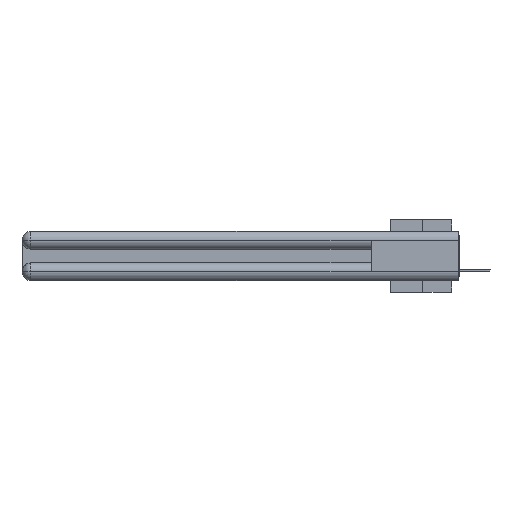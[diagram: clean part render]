
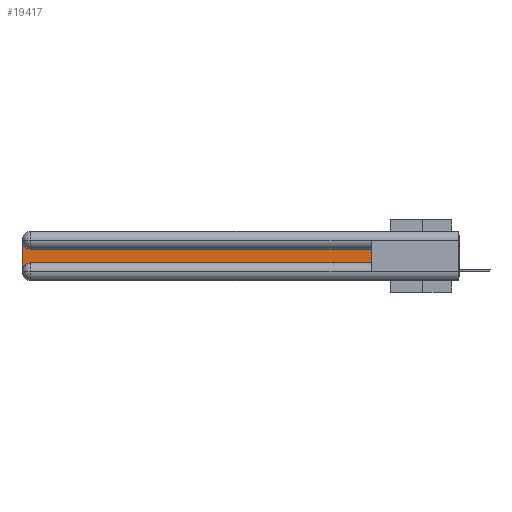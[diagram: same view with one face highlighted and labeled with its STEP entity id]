
A CAD part, left-side view. The second image highlights one B-rep face of the part: STEP entity #19417.
In plain terms, the highlighted planar face has unit normal (-1, 0, 0).
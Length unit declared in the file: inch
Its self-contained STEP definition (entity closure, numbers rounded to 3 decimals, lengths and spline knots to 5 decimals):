
#519 = FACE_OUTER_BOUND ( 'NONE', #23356, .T. ) ;
#742 = CARTESIAN_POINT ( 'NONE',  ( 0.075, 2.94, -0.2175 ) ) ;
#866 = EDGE_CURVE ( 'NONE', #18153, #22871, #3289, .T. ) ;
#1136 = VERTEX_POINT ( 'NONE', #16939 ) ;
#1238 = EDGE_CURVE ( 'NONE', #1136, #14046, #23736, .T. ) ;
#2180 = CARTESIAN_POINT ( 'NONE',  ( 0.075, 0.6, -0.2175 ) ) ;
#2908 = ORIENTED_EDGE ( 'NONE', *, *, #7068, .T. ) ;
#3167 = LINE ( 'NONE', #16044, #13963 ) ;
#3289 = LINE ( 'NONE', #4976, #29496 ) ;
#3975 = CARTESIAN_POINT ( 'NONE',  ( 0.075, 3., -0.0625 ) ) ;
#4450 = VERTEX_POINT ( 'NONE', #3975 ) ;
#4482 = VECTOR ( 'NONE', #19351, 39.37008 ) ;
#4976 = CARTESIAN_POINT ( 'NONE',  ( 0.075, 0.6, -0.2175 ) ) ;
#5127 = CARTESIAN_POINT ( 'NONE',  ( 0.075, 2.94, -0.1225 ) ) ;
#5492 = ORIENTED_EDGE ( 'NONE', *, *, #1238, .T. ) ;
#6933 = ORIENTED_EDGE ( 'NONE', *, *, #866, .T. ) ;
#7068 = EDGE_CURVE ( 'NONE', #4450, #1136, #25303, .T. ) ;
#7248 = AXIS2_PLACEMENT_3D ( 'NONE', #15810, #22698, #15716 ) ;
#7595 = DIRECTION ( 'NONE',  ( 0., -1., 0. ) ) ;
#10339 = CARTESIAN_POINT ( 'NONE',  ( 0.075, 3., -0.2175 ) ) ;
#10542 = CARTESIAN_POINT ( 'NONE',  ( 0.075, 0.6, -0.1225 ) ) ;
#10583 = VERTEX_POINT ( 'NONE', #5127 ) ;
#11145 = EDGE_CURVE ( 'NONE', #14046, #18153, #12526, .T. ) ;
#12526 = LINE ( 'NONE', #19443, #23641 ) ;
#12702 = AXIS2_PLACEMENT_3D ( 'NONE', #24027, #14924, #15028 ) ;
#13338 = CIRCLE ( 'NONE', #24314, 0.06 ) ;
#13963 = VECTOR ( 'NONE', #18340, 39.37008 ) ;
#14046 = VERTEX_POINT ( 'NONE', #742 ) ;
#14924 = DIRECTION ( 'NONE',  ( 1., 0., 0. ) ) ;
#15028 = DIRECTION ( 'NONE',  ( 0., 0., -1. ) ) ;
#15716 = DIRECTION ( 'NONE',  ( 0., 0., -1. ) ) ;
#15810 = CARTESIAN_POINT ( 'NONE',  ( 0.075, 3., -0.1225 ) ) ;
#16044 = CARTESIAN_POINT ( 'NONE',  ( 0.075, 0.6, -0.1225 ) ) ;
#16777 = EDGE_CURVE ( 'NONE', #10583, #4450, #13338, .T. ) ;
#16939 = CARTESIAN_POINT ( 'NONE',  ( 0.075, 3., -0.2775 ) ) ;
#17847 = ORIENTED_EDGE ( 'NONE', *, *, #16777, .T. ) ;
#18153 = VERTEX_POINT ( 'NONE', #2180 ) ;
#18340 = DIRECTION ( 'NONE',  ( 0., 1., 0. ) ) ;
#19351 = DIRECTION ( 'NONE',  ( 0., 0., -1. ) ) ;
#19417 = ADVANCED_FACE ( 'NONE', ( #519 ), #27223, .F. ) ;
#19443 = CARTESIAN_POINT ( 'NONE',  ( 0.075, 0.6, -0.2175 ) ) ;
#22698 = DIRECTION ( 'NONE',  ( 1., 0., 0. ) ) ;
#22871 = VERTEX_POINT ( 'NONE', #10542 ) ;
#22933 = DIRECTION ( 'NONE',  ( 0., 0., 1. ) ) ;
#23356 = EDGE_LOOP ( 'NONE', ( #26018, #17847, #2908, #5492, #26583, #6933 ) ) ;
#23453 = CARTESIAN_POINT ( 'NONE',  ( 0.075, 2.94, -0.0625 ) ) ;
#23641 = VECTOR ( 'NONE', #7595, 39.37008 ) ;
#23736 = CIRCLE ( 'NONE', #12702, 0.06 ) ;
#24027 = CARTESIAN_POINT ( 'NONE',  ( 0.075, 2.94, -0.2775 ) ) ;
#24314 = AXIS2_PLACEMENT_3D ( 'NONE', #23453, #25757, #25659 ) ;
#25303 = LINE ( 'NONE', #10339, #4482 ) ;
#25659 = DIRECTION ( 'NONE',  ( 0., 0., -1. ) ) ;
#25757 = DIRECTION ( 'NONE',  ( 1., 0., 0. ) ) ;
#26018 = ORIENTED_EDGE ( 'NONE', *, *, #28001, .T. ) ;
#26583 = ORIENTED_EDGE ( 'NONE', *, *, #11145, .T. ) ;
#27223 = PLANE ( 'NONE',  #7248 ) ;
#28001 = EDGE_CURVE ( 'NONE', #22871, #10583, #3167, .T. ) ;
#29496 = VECTOR ( 'NONE', #22933, 39.37008 ) ;
